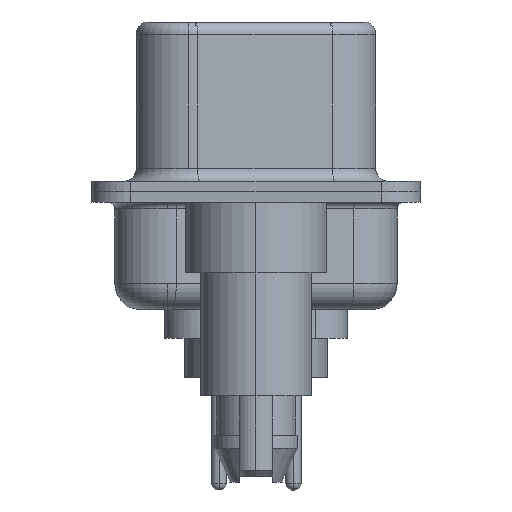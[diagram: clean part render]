
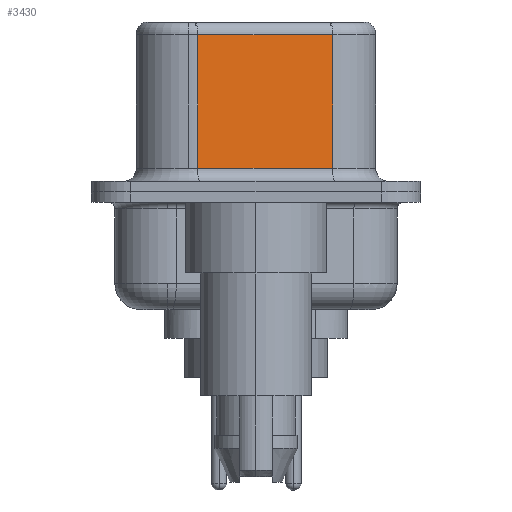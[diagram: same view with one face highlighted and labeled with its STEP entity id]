
A CAD part, left-side view. The second image highlights one B-rep face of the part: STEP entity #3430.
In plain terms, the highlighted planar face has unit normal (-0.985, -0.174, 0).
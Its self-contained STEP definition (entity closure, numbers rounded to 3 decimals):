
#5 = VERTEX_POINT ( 'NONE', #20409 ) ;
#203 = AXIS2_PLACEMENT_3D ( 'NONE', #15737, #16063, #15925 ) ;
#548 = DIRECTION ( 'NONE',  ( 0., 0., -1. ) ) ;
#626 = ORIENTED_EDGE ( 'NONE', *, *, #6462, .F. ) ;
#1253 = VECTOR ( 'NONE', #10423, 1000. ) ;
#1340 = EDGE_LOOP ( 'NONE', ( #626, #1762, #5330, #10267 ) ) ;
#1762 = ORIENTED_EDGE ( 'NONE', *, *, #18839, .T. ) ;
#3304 = LINE ( 'NONE', #11869, #22583 ) ;
#3430 = ADVANCED_FACE ( 'NONE', ( #10831 ), #18749, .F. ) ;
#3873 = CARTESIAN_POINT ( 'NONE',  ( 4.58, -2.927, 6.52 ) ) ;
#4359 = CARTESIAN_POINT ( 'NONE',  ( 3.67, 2.233, 0.9 ) ) ;
#5330 = ORIENTED_EDGE ( 'NONE', *, *, #15434, .T. ) ;
#5720 = VECTOR ( 'NONE', #18741, 1000. ) ;
#6324 = CARTESIAN_POINT ( 'NONE',  ( 4.58, -2.927, 6.02 ) ) ;
#6325 = LINE ( 'NONE', #7567, #5720 ) ;
#6374 = VECTOR ( 'NONE', #12236, 1000. ) ;
#6462 = EDGE_CURVE ( 'NONE', #19110, #10328, #21144, .T. ) ;
#7567 = CARTESIAN_POINT ( 'NONE',  ( 4.58, -2.927, 6.02 ) ) ;
#7793 = CARTESIAN_POINT ( 'NONE',  ( 4.58, -2.927, 0.9 ) ) ;
#10267 = ORIENTED_EDGE ( 'NONE', *, *, #16728, .T. ) ;
#10328 = VERTEX_POINT ( 'NONE', #7793 ) ;
#10423 = DIRECTION ( 'NONE',  ( 0., 0., -1. ) ) ;
#10831 = FACE_OUTER_BOUND ( 'NONE', #1340, .T. ) ;
#11869 = CARTESIAN_POINT ( 'NONE',  ( 3.67, 2.233, 6.52 ) ) ;
#12236 = DIRECTION ( 'NONE',  ( 0.174, -0.985, 0. ) ) ;
#15434 = EDGE_CURVE ( 'NONE', #5, #16025, #3304, .T. ) ;
#15737 = CARTESIAN_POINT ( 'NONE',  ( 4.58, -2.927, 6.52 ) ) ;
#15925 = DIRECTION ( 'NONE',  ( -0.174, 0.985, 0. ) ) ;
#16025 = VERTEX_POINT ( 'NONE', #4359 ) ;
#16063 = DIRECTION ( 'NONE',  ( 0.985, 0.174, 0. ) ) ;
#16325 = LINE ( 'NONE', #23304, #6374 ) ;
#16728 = EDGE_CURVE ( 'NONE', #16025, #10328, #16325, .T. ) ;
#18741 = DIRECTION ( 'NONE',  ( -0.174, 0.985, 0. ) ) ;
#18749 = PLANE ( 'NONE',  #203 ) ;
#18839 = EDGE_CURVE ( 'NONE', #19110, #5, #6325, .T. ) ;
#19110 = VERTEX_POINT ( 'NONE', #6324 ) ;
#20409 = CARTESIAN_POINT ( 'NONE',  ( 3.67, 2.233, 6.02 ) ) ;
#21144 = LINE ( 'NONE', #3873, #1253 ) ;
#22583 = VECTOR ( 'NONE', #548, 1000. ) ;
#23304 = CARTESIAN_POINT ( 'NONE',  ( 4.58, -2.927, 0.9 ) ) ;
